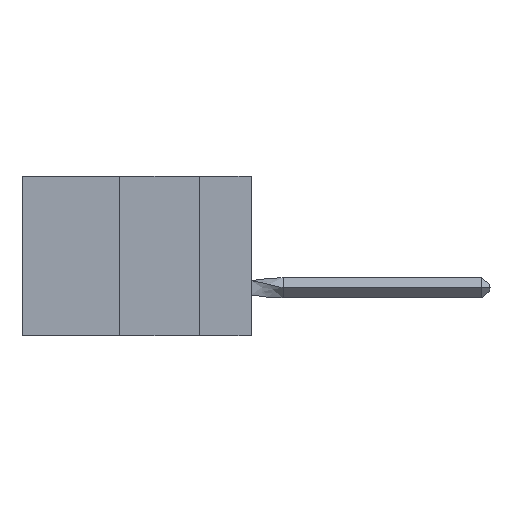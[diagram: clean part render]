
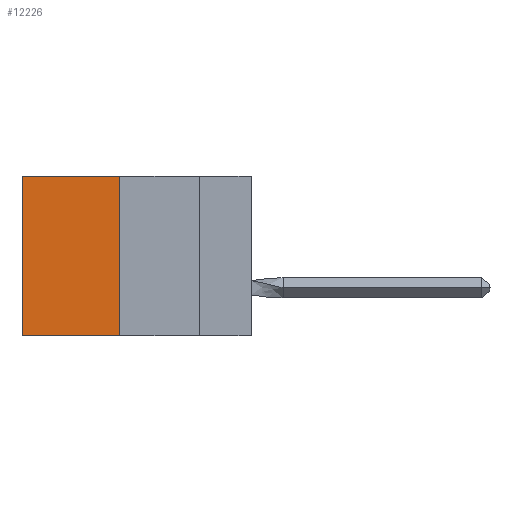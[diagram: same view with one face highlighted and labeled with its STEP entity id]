
A CAD part, left-side view. The second image highlights one B-rep face of the part: STEP entity #12226.
In plain terms, the highlighted planar face has unit normal (-1, 0, 0).
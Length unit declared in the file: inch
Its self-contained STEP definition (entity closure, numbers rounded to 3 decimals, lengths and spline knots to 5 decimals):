
#22 = CARTESIAN_POINT ( 'NONE',  ( 0.305, 0.72, -0.5 ) ) ;
#977 = VERTEX_POINT ( 'NONE', #22 ) ;
#1027 = FACE_OUTER_BOUND ( 'NONE', #5406, .T. ) ;
#1171 = LINE ( 'NONE', #8748, #2135 ) ;
#1293 = LINE ( 'NONE', #19057, #5461 ) ;
#1870 = CARTESIAN_POINT ( 'NONE',  ( 0.305, 0.72, -0.5 ) ) ;
#2135 = VECTOR ( 'NONE', #4449, 39.37008 ) ;
#2556 = EDGE_CURVE ( 'NONE', #12514, #977, #1293, .T. ) ;
#3040 = CARTESIAN_POINT ( 'NONE',  ( 0.305, 0.72, 0. ) ) ;
#3861 = DIRECTION ( 'NONE',  ( 0., 0., -1. ) ) ;
#4292 = LINE ( 'NONE', #6140, #11039 ) ;
#4377 = VERTEX_POINT ( 'NONE', #3040 ) ;
#4449 = DIRECTION ( 'NONE',  ( 0., 0., -1. ) ) ;
#4522 = PLANE ( 'NONE',  #18724 ) ;
#4771 = EDGE_CURVE ( 'NONE', #9034, #12514, #1171, .T. ) ;
#5406 = EDGE_LOOP ( 'NONE', ( #17676, #6404, #17363, #7860 ) ) ;
#5461 = VECTOR ( 'NONE', #14805, 39.37008 ) ;
#6140 = CARTESIAN_POINT ( 'NONE',  ( 0.305, 0.413, 0. ) ) ;
#6371 = EDGE_CURVE ( 'NONE', #9034, #4377, #4292, .T. ) ;
#6404 = ORIENTED_EDGE ( 'NONE', *, *, #2556, .F. ) ;
#7860 = ORIENTED_EDGE ( 'NONE', *, *, #6371, .T. ) ;
#8748 = CARTESIAN_POINT ( 'NONE',  ( 0.305, 0.413, -0.5 ) ) ;
#9034 = VERTEX_POINT ( 'NONE', #21110 ) ;
#10346 = DIRECTION ( 'NONE',  ( 0., 1., 0. ) ) ;
#11039 = VECTOR ( 'NONE', #10346, 39.37008 ) ;
#11760 = CARTESIAN_POINT ( 'NONE',  ( 0.305, 0.413, -0.5 ) ) ;
#12226 = ADVANCED_FACE ( 'NONE', ( #1027 ), #4522, .F. ) ;
#12514 = VERTEX_POINT ( 'NONE', #11760 ) ;
#14805 = DIRECTION ( 'NONE',  ( 0., 1., 0. ) ) ;
#17363 = ORIENTED_EDGE ( 'NONE', *, *, #4771, .F. ) ;
#17676 = ORIENTED_EDGE ( 'NONE', *, *, #23411, .T. ) ;
#18724 = AXIS2_PLACEMENT_3D ( 'NONE', #23006, #18826, #20856 ) ;
#18826 = DIRECTION ( 'NONE',  ( 1., 0., 0. ) ) ;
#19057 = CARTESIAN_POINT ( 'NONE',  ( 0.305, 0.413, -0.5 ) ) ;
#20170 = LINE ( 'NONE', #1870, #23035 ) ;
#20856 = DIRECTION ( 'NONE',  ( 0., 0., -1. ) ) ;
#21110 = CARTESIAN_POINT ( 'NONE',  ( 0.305, 0.413, 0. ) ) ;
#23006 = CARTESIAN_POINT ( 'NONE',  ( 0.305, 0.413, -0.5 ) ) ;
#23035 = VECTOR ( 'NONE', #3861, 39.37008 ) ;
#23411 = EDGE_CURVE ( 'NONE', #4377, #977, #20170, .T. ) ;
